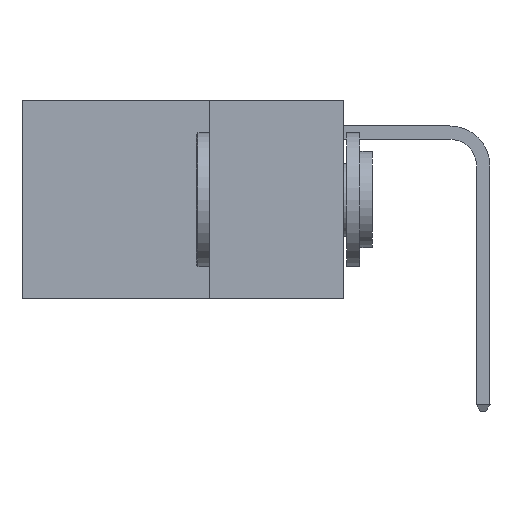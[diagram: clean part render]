
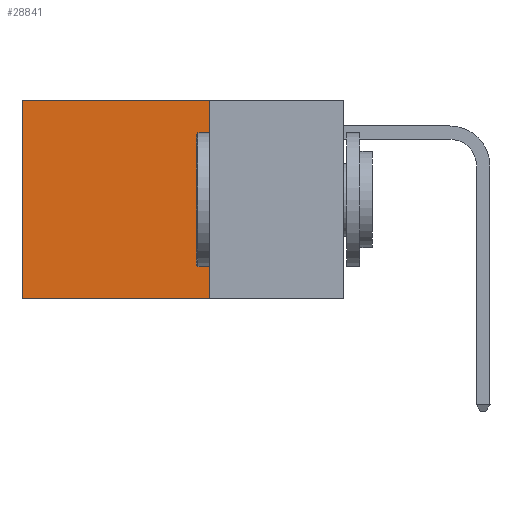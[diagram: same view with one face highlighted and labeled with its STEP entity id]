
A CAD part, left-side view. The second image highlights one B-rep face of the part: STEP entity #28841.
In plain terms, the highlighted planar face has unit normal (-1, 0, 0).
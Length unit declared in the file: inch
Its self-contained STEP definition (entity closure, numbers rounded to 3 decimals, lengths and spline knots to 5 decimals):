
#885 = CARTESIAN_POINT ( 'NONE',  ( 0.2625, 0.25, 0. ) ) ;
#2235 = DIRECTION ( 'NONE',  ( 0., 0., -1. ) ) ;
#3758 = VECTOR ( 'NONE', #2235, 39.37008 ) ;
#3785 = VERTEX_POINT ( 'NONE', #19183 ) ;
#4003 = CARTESIAN_POINT ( 'NONE',  ( 0.2625, 0.25, 0. ) ) ;
#4058 = ORIENTED_EDGE ( 'NONE', *, *, #27711, .F. ) ;
#4918 = VERTEX_POINT ( 'NONE', #20816 ) ;
#5382 = ORIENTED_EDGE ( 'NONE', *, *, #15029, .T. ) ;
#5434 = LINE ( 'NONE', #885, #21194 ) ;
#6108 = FACE_OUTER_BOUND ( 'NONE', #11389, .T. ) ;
#6658 = DIRECTION ( 'NONE',  ( 0., 0., -1. ) ) ;
#7720 = DIRECTION ( 'NONE',  ( 0., 1., 0. ) ) ;
#11224 = ORIENTED_EDGE ( 'NONE', *, *, #16030, .T. ) ;
#11389 = EDGE_LOOP ( 'NONE', ( #11224, #4058, #19131, #5382 ) ) ;
#11920 = LINE ( 'NONE', #13866, #15814 ) ;
#12857 = CARTESIAN_POINT ( 'NONE',  ( 0.2625, 0.25, 0. ) ) ;
#13253 = VERTEX_POINT ( 'NONE', #16226 ) ;
#13866 = CARTESIAN_POINT ( 'NONE',  ( 0.2625, 0.25, -0.37 ) ) ;
#15029 = EDGE_CURVE ( 'NONE', #23028, #13253, #5434, .T. ) ;
#15814 = VECTOR ( 'NONE', #21178, 39.37008 ) ;
#16030 = EDGE_CURVE ( 'NONE', #13253, #3785, #17767, .T. ) ;
#16226 = CARTESIAN_POINT ( 'NONE',  ( 0.2625, 0.6, 0. ) ) ;
#16714 = EDGE_CURVE ( 'NONE', #23028, #4918, #30002, .T. ) ;
#17767 = LINE ( 'NONE', #27127, #19735 ) ;
#18351 = CARTESIAN_POINT ( 'NONE',  ( 0.2625, 0.25, 0. ) ) ;
#19131 = ORIENTED_EDGE ( 'NONE', *, *, #16714, .F. ) ;
#19183 = CARTESIAN_POINT ( 'NONE',  ( 0.2625, 0.6, -0.37 ) ) ;
#19735 = VECTOR ( 'NONE', #6658, 39.37008 ) ;
#20816 = CARTESIAN_POINT ( 'NONE',  ( 0.2625, 0.25, -0.37 ) ) ;
#21178 = DIRECTION ( 'NONE',  ( 0., 1., 0. ) ) ;
#21194 = VECTOR ( 'NONE', #7720, 39.37008 ) ;
#21844 = DIRECTION ( 'NONE',  ( 1., 0., 0. ) ) ;
#23028 = VERTEX_POINT ( 'NONE', #4003 ) ;
#24432 = DIRECTION ( 'NONE',  ( 0., 0., -1. ) ) ;
#26900 = PLANE ( 'NONE',  #28693 ) ;
#27127 = CARTESIAN_POINT ( 'NONE',  ( 0.2625, 0.6, 0. ) ) ;
#27711 = EDGE_CURVE ( 'NONE', #4918, #3785, #11920, .T. ) ;
#28693 = AXIS2_PLACEMENT_3D ( 'NONE', #12857, #21844, #24432 ) ;
#28841 = ADVANCED_FACE ( 'NONE', ( #6108 ), #26900, .F. ) ;
#30002 = LINE ( 'NONE', #18351, #3758 ) ;
